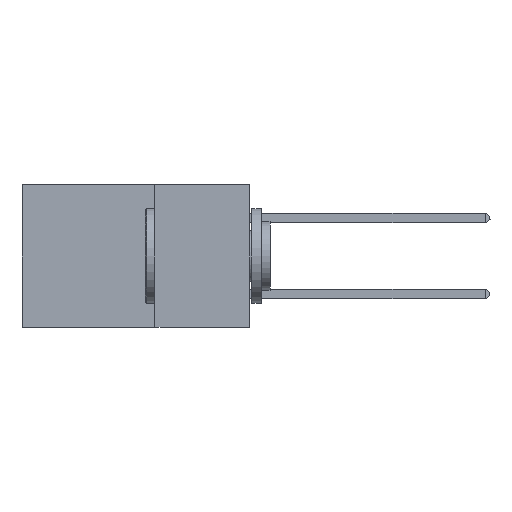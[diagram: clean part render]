
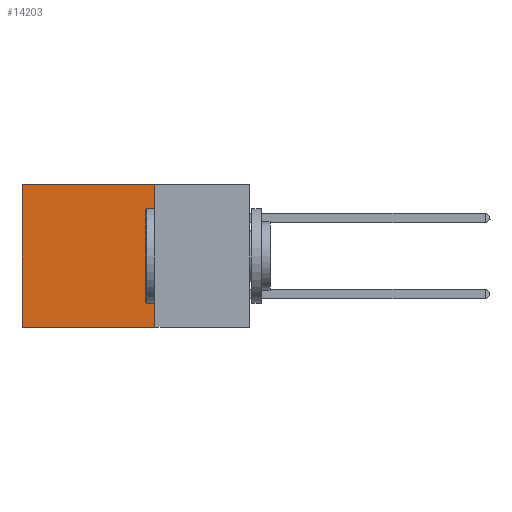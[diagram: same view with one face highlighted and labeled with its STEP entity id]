
A CAD part, left-side view. The second image highlights one B-rep face of the part: STEP entity #14203.
In plain terms, the highlighted planar face has unit normal (-1, 0, 0).
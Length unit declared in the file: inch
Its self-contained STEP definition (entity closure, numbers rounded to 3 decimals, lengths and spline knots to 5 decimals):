
#338 = VECTOR ( 'NONE', #7383, 39.37008 ) ;
#596 = DIRECTION ( 'NONE',  ( 0., 1., 0. ) ) ;
#1657 = DIRECTION ( 'NONE',  ( 1., 0., 0. ) ) ;
#2435 = VECTOR ( 'NONE', #14208, 39.37008 ) ;
#2466 = PLANE ( 'NONE',  #6852 ) ;
#2954 = LINE ( 'NONE', #10060, #11714 ) ;
#3513 = EDGE_CURVE ( 'NONE', #6097, #12036, #2954, .T. ) ;
#3617 = FACE_OUTER_BOUND ( 'NONE', #5497, .T. ) ;
#3752 = CARTESIAN_POINT ( 'NONE',  ( 0.2875, 0.6, 0. ) ) ;
#4214 = VERTEX_POINT ( 'NONE', #12162 ) ;
#5267 = CARTESIAN_POINT ( 'NONE',  ( 0.2875, 0.25, -0.375 ) ) ;
#5478 = DIRECTION ( 'NONE',  ( 0., 1., 0. ) ) ;
#5497 = EDGE_LOOP ( 'NONE', ( #10257, #11430, #6962, #10399 ) ) ;
#6071 = DIRECTION ( 'NONE',  ( 0., 0., -1. ) ) ;
#6097 = VERTEX_POINT ( 'NONE', #13100 ) ;
#6357 = LINE ( 'NONE', #5267, #338 ) ;
#6852 = AXIS2_PLACEMENT_3D ( 'NONE', #9438, #1657, #6071 ) ;
#6962 = ORIENTED_EDGE ( 'NONE', *, *, #13163, .F. ) ;
#7383 = DIRECTION ( 'NONE',  ( 0., 0., -1. ) ) ;
#8109 = CARTESIAN_POINT ( 'NONE',  ( 0.2875, 0.6, -0.375 ) ) ;
#8828 = VERTEX_POINT ( 'NONE', #3752 ) ;
#9438 = CARTESIAN_POINT ( 'NONE',  ( 0.2875, 0.25, -0.375 ) ) ;
#10060 = CARTESIAN_POINT ( 'NONE',  ( 0.2875, 0.25, -0.375 ) ) ;
#10257 = ORIENTED_EDGE ( 'NONE', *, *, #13339, .T. ) ;
#10399 = ORIENTED_EDGE ( 'NONE', *, *, #12694, .T. ) ;
#10568 = LINE ( 'NONE', #13967, #12407 ) ;
#11430 = ORIENTED_EDGE ( 'NONE', *, *, #3513, .F. ) ;
#11714 = VECTOR ( 'NONE', #5478, 39.37008 ) ;
#12036 = VERTEX_POINT ( 'NONE', #8109 ) ;
#12111 = CARTESIAN_POINT ( 'NONE',  ( 0.2875, 0.6, -0.375 ) ) ;
#12162 = CARTESIAN_POINT ( 'NONE',  ( 0.2875, 0.25, 0. ) ) ;
#12407 = VECTOR ( 'NONE', #596, 39.37008 ) ;
#12694 = EDGE_CURVE ( 'NONE', #4214, #8828, #10568, .T. ) ;
#13100 = CARTESIAN_POINT ( 'NONE',  ( 0.2875, 0.25, -0.375 ) ) ;
#13163 = EDGE_CURVE ( 'NONE', #4214, #6097, #6357, .T. ) ;
#13339 = EDGE_CURVE ( 'NONE', #8828, #12036, #13412, .T. ) ;
#13412 = LINE ( 'NONE', #12111, #2435 ) ;
#13967 = CARTESIAN_POINT ( 'NONE',  ( 0.2875, 0.25, 0. ) ) ;
#14203 = ADVANCED_FACE ( 'NONE', ( #3617 ), #2466, .F. ) ;
#14208 = DIRECTION ( 'NONE',  ( 0., 0., -1. ) ) ;
